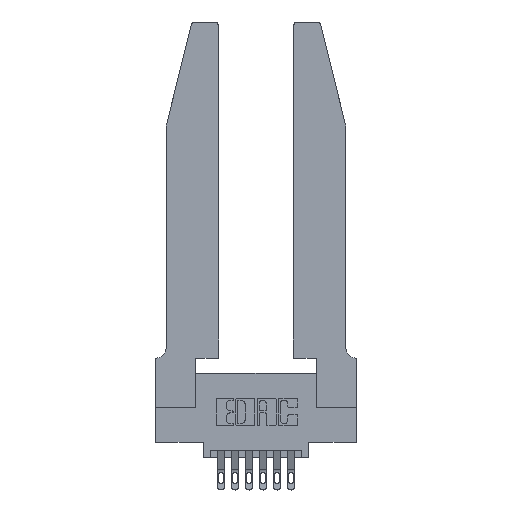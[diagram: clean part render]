
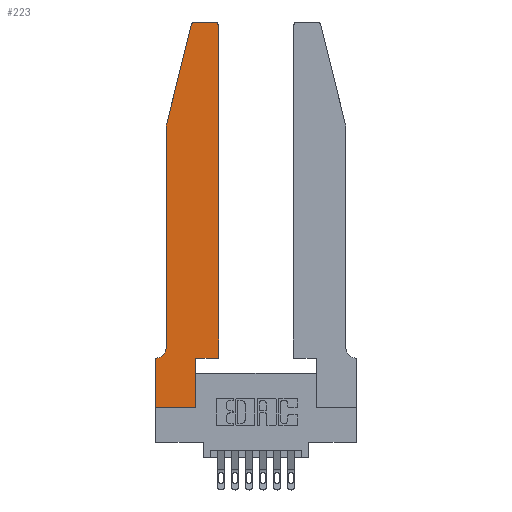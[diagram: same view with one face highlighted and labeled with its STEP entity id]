
A CAD part, top view. The second image highlights one B-rep face of the part: STEP entity #223.
In plain terms, the highlighted planar face has unit normal (0, 0, 1).
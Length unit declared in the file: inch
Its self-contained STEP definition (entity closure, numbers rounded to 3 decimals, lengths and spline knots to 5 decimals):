
#41 = VERTEX_POINT ( 'NONE', #7402 ) ;
#103 = CIRCLE ( 'NONE', #11234, 0.03 ) ;
#223 = ADVANCED_FACE ( 'NONE', ( #5406 ), #6758, .T. ) ;
#454 = ORIENTED_EDGE ( 'NONE', *, *, #10786, .T. ) ;
#505 = DIRECTION ( 'NONE',  ( 1., 0., 0. ) ) ;
#540 = CARTESIAN_POINT ( 'NONE',  ( 0.284, 2.75, 0.37 ) ) ;
#731 = EDGE_CURVE ( 'NONE', #12710, #2707, #8676, .T. ) ;
#904 = VERTEX_POINT ( 'NONE', #2288 ) ;
#1371 = CIRCLE ( 'NONE', #10614, 0.07 ) ;
#1616 = AXIS2_PLACEMENT_3D ( 'NONE', #6676, #14326, #7792 ) ;
#1822 = CARTESIAN_POINT ( 'NONE',  ( 0., 0., 0.37 ) ) ;
#1921 = EDGE_CURVE ( 'NONE', #11187, #9045, #5370, .T. ) ;
#1953 = CARTESIAN_POINT ( 'NONE',  ( 0.4505, 0.35, 0.37 ) ) ;
#2068 = DIRECTION ( 'NONE',  ( 0., -1., 0. ) ) ;
#2247 = CARTESIAN_POINT ( 'NONE',  ( 0.4205, 2.75, 0.37 ) ) ;
#2288 = CARTESIAN_POINT ( 'NONE',  ( 0.2865, 0., 0.37 ) ) ;
#2311 = DIRECTION ( 'NONE',  ( -1., 0., 0. ) ) ;
#2707 = VERTEX_POINT ( 'NONE', #540 ) ;
#2737 = VERTEX_POINT ( 'NONE', #10518 ) ;
#3043 = VECTOR ( 'NONE', #4813, 39.37008 ) ;
#3208 = DIRECTION ( 'NONE',  ( 1., 0., 0. ) ) ;
#3364 = LINE ( 'NONE', #11441, #11849 ) ;
#3466 = CARTESIAN_POINT ( 'NONE',  ( 0., 0.35, 0.37 ) ) ;
#4009 = DIRECTION ( 'NONE',  ( 0., 0., -1. ) ) ;
#4163 = ORIENTED_EDGE ( 'NONE', *, *, #10751, .T. ) ;
#4463 = ORIENTED_EDGE ( 'NONE', *, *, #1921, .T. ) ;
#4498 = VECTOR ( 'NONE', #505, 39.37008 ) ;
#4645 = LINE ( 'NONE', #9004, #10161 ) ;
#4654 = VECTOR ( 'NONE', #4937, 39.37008 ) ;
#4744 = ORIENTED_EDGE ( 'NONE', *, *, #13613, .T. ) ;
#4813 = DIRECTION ( 'NONE',  ( -1., 0., 0. ) ) ;
#4937 = DIRECTION ( 'NONE',  ( 0., -1., 0. ) ) ;
#5062 = AXIS2_PLACEMENT_3D ( 'NONE', #3466, #6741, #6275 ) ;
#5180 = CARTESIAN_POINT ( 'NONE',  ( 0.0755, 2., 0.37 ) ) ;
#5366 = CARTESIAN_POINT ( 'NONE',  ( 0.2865, 0.35, 0.37 ) ) ;
#5370 = LINE ( 'NONE', #14428, #4654 ) ;
#5400 = ORIENTED_EDGE ( 'NONE', *, *, #10252, .T. ) ;
#5406 = FACE_OUTER_BOUND ( 'NONE', #12767, .T. ) ;
#5477 = EDGE_CURVE ( 'NONE', #8047, #12710, #103, .T. ) ;
#5603 = ORIENTED_EDGE ( 'NONE', *, *, #14688, .T. ) ;
#5674 = VERTEX_POINT ( 'NONE', #12604 ) ;
#5686 = DIRECTION ( 'NONE',  ( -0.239, -0.971, 0. ) ) ;
#5776 = LINE ( 'NONE', #14548, #8346 ) ;
#5781 = CARTESIAN_POINT ( 'NONE',  ( 0.2605, 2.75, 0.37 ) ) ;
#5919 = CARTESIAN_POINT ( 'NONE',  ( 0.2865, 0.35, 0.37 ) ) ;
#5921 = CARTESIAN_POINT ( 'NONE',  ( 0.4505, 2.72, 0.37 ) ) ;
#6275 = DIRECTION ( 'NONE',  ( 1., 0., 0. ) ) ;
#6381 = ORIENTED_EDGE ( 'NONE', *, *, #5477, .T. ) ;
#6676 = CARTESIAN_POINT ( 'NONE',  ( 0.284, 2.72, 0.37 ) ) ;
#6741 = DIRECTION ( 'NONE',  ( 0., 0., 1. ) ) ;
#6758 = PLANE ( 'NONE',  #5062 ) ;
#6895 = DIRECTION ( 'NONE',  ( 0., 0., 1. ) ) ;
#7019 = EDGE_CURVE ( 'NONE', #9045, #2737, #1371, .T. ) ;
#7402 = CARTESIAN_POINT ( 'NONE',  ( 0.4505, 0.35, 0.37 ) ) ;
#7426 = LINE ( 'NONE', #5366, #9672 ) ;
#7630 = CARTESIAN_POINT ( 'NONE',  ( 0.25487, 2.72718, 0.37 ) ) ;
#7792 = DIRECTION ( 'NONE',  ( 1., 0., 0. ) ) ;
#7800 = LINE ( 'NONE', #1822, #4498 ) ;
#8047 = VERTEX_POINT ( 'NONE', #5921 ) ;
#8346 = VECTOR ( 'NONE', #2311, 39.37008 ) ;
#8676 = LINE ( 'NONE', #5781, #3043 ) ;
#8689 = LINE ( 'NONE', #1953, #14132 ) ;
#9004 = CARTESIAN_POINT ( 'NONE',  ( 0., 0., 0.37 ) ) ;
#9014 = CARTESIAN_POINT ( 'NONE',  ( 0.0755, 2., 0.37 ) ) ;
#9045 = VERTEX_POINT ( 'NONE', #13111 ) ;
#9412 = VECTOR ( 'NONE', #5686, 39.37008 ) ;
#9672 = VECTOR ( 'NONE', #11907, 39.37008 ) ;
#9762 = ORIENTED_EDGE ( 'NONE', *, *, #11960, .T. ) ;
#9858 = ORIENTED_EDGE ( 'NONE', *, *, #12630, .T. ) ;
#9896 = ORIENTED_EDGE ( 'NONE', *, *, #10299, .T. ) ;
#9922 = CARTESIAN_POINT ( 'NONE',  ( 0., 0., 0.37 ) ) ;
#10161 = VECTOR ( 'NONE', #2068, 39.37008 ) ;
#10252 = EDGE_CURVE ( 'NONE', #14305, #11187, #11921, .T. ) ;
#10299 = EDGE_CURVE ( 'NONE', #2737, #5674, #5776, .T. ) ;
#10322 = ORIENTED_EDGE ( 'NONE', *, *, #731, .T. ) ;
#10518 = CARTESIAN_POINT ( 'NONE',  ( 0.0055, 0.35, 0.37 ) ) ;
#10614 = AXIS2_PLACEMENT_3D ( 'NONE', #10640, #4009, #11710 ) ;
#10640 = CARTESIAN_POINT ( 'NONE',  ( 0.0055, 0.42, 0.37 ) ) ;
#10751 = EDGE_CURVE ( 'NONE', #12728, #41, #8689, .T. ) ;
#10786 = EDGE_CURVE ( 'NONE', #2707, #14305, #10895, .T. ) ;
#10895 = CIRCLE ( 'NONE', #1616, 0.03 ) ;
#11187 = VERTEX_POINT ( 'NONE', #5180 ) ;
#11234 = AXIS2_PLACEMENT_3D ( 'NONE', #13426, #6895, #14574 ) ;
#11441 = CARTESIAN_POINT ( 'NONE',  ( 0.4505, 0.35, 0.37 ) ) ;
#11504 = ORIENTED_EDGE ( 'NONE', *, *, #7019, .T. ) ;
#11710 = DIRECTION ( 'NONE',  ( -1., 0., 0. ) ) ;
#11849 = VECTOR ( 'NONE', #12559, 39.37008 ) ;
#11907 = DIRECTION ( 'NONE',  ( 0., 1., 0. ) ) ;
#11921 = LINE ( 'NONE', #9014, #9412 ) ;
#11960 = EDGE_CURVE ( 'NONE', #904, #12728, #7426, .T. ) ;
#12559 = DIRECTION ( 'NONE',  ( 0., 1., 0. ) ) ;
#12604 = CARTESIAN_POINT ( 'NONE',  ( 0., 0.35, 0.37 ) ) ;
#12630 = EDGE_CURVE ( 'NONE', #5674, #13663, #4645, .T. ) ;
#12710 = VERTEX_POINT ( 'NONE', #2247 ) ;
#12728 = VERTEX_POINT ( 'NONE', #5919 ) ;
#12767 = EDGE_LOOP ( 'NONE', ( #10322, #454, #5400, #4463, #11504, #9896, #9858, #4744, #9762, #4163, #5603, #6381 ) ) ;
#13111 = CARTESIAN_POINT ( 'NONE',  ( 0.0755, 0.42, 0.37 ) ) ;
#13426 = CARTESIAN_POINT ( 'NONE',  ( 0.4205, 2.72, 0.37 ) ) ;
#13613 = EDGE_CURVE ( 'NONE', #13663, #904, #7800, .T. ) ;
#13663 = VERTEX_POINT ( 'NONE', #9922 ) ;
#14132 = VECTOR ( 'NONE', #3208, 39.37008 ) ;
#14305 = VERTEX_POINT ( 'NONE', #7630 ) ;
#14326 = DIRECTION ( 'NONE',  ( 0., 0., 1. ) ) ;
#14428 = CARTESIAN_POINT ( 'NONE',  ( 0.0755, 2., 0.37 ) ) ;
#14548 = CARTESIAN_POINT ( 'NONE',  ( 0.0755, 0.35, 0.37 ) ) ;
#14574 = DIRECTION ( 'NONE',  ( 1., 0., 0. ) ) ;
#14688 = EDGE_CURVE ( 'NONE', #41, #8047, #3364, .T. ) ;
